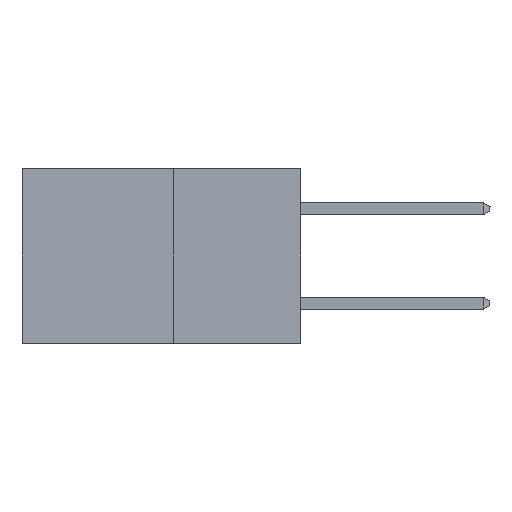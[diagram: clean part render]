
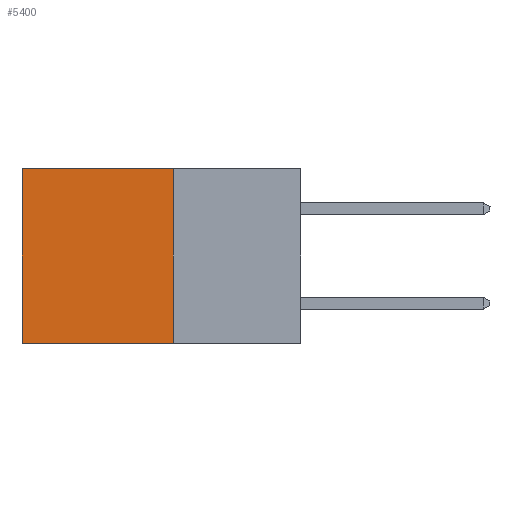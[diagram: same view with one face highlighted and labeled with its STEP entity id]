
A CAD part, left-side view. The second image highlights one B-rep face of the part: STEP entity #5400.
In plain terms, the highlighted planar face has unit normal (-1, 0, 0).
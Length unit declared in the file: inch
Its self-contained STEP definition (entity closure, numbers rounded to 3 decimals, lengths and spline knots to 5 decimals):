
#176 = CARTESIAN_POINT ( 'NONE',  ( 0.277, 0.27, -0.37 ) ) ;
#499 = CARTESIAN_POINT ( 'NONE',  ( 0.277, 0.59, -0.37 ) ) ;
#504 = FACE_OUTER_BOUND ( 'NONE', #11642, .T. ) ;
#892 = VECTOR ( 'NONE', #5699, 39.37008 ) ;
#1214 = VECTOR ( 'NONE', #12525, 39.37008 ) ;
#1572 = EDGE_CURVE ( 'NONE', #10851, #7207, #12171, .T. ) ;
#3573 = LINE ( 'NONE', #499, #892 ) ;
#3858 = CARTESIAN_POINT ( 'NONE',  ( 0.277, 0.27, -0.37 ) ) ;
#4150 = EDGE_CURVE ( 'NONE', #10851, #6409, #7095, .T. ) ;
#4247 = DIRECTION ( 'NONE',  ( 1., 0., 0. ) ) ;
#4442 = CARTESIAN_POINT ( 'NONE',  ( 0.277, 0.27, -0.37 ) ) ;
#4604 = DIRECTION ( 'NONE',  ( 0., 1., 0. ) ) ;
#4694 = EDGE_CURVE ( 'NONE', #6409, #11805, #8443, .T. ) ;
#4986 = ORIENTED_EDGE ( 'NONE', *, *, #4694, .F. ) ;
#5400 = ADVANCED_FACE ( 'NONE', ( #504 ), #7742, .F. ) ;
#5445 = CARTESIAN_POINT ( 'NONE',  ( 0.277, 0.59, -0.37 ) ) ;
#5451 = DIRECTION ( 'NONE',  ( 0., 0., -1. ) ) ;
#5509 = VECTOR ( 'NONE', #4604, 39.37008 ) ;
#5699 = DIRECTION ( 'NONE',  ( 0., 0., -1. ) ) ;
#6409 = VERTEX_POINT ( 'NONE', #3858 ) ;
#6990 = ORIENTED_EDGE ( 'NONE', *, *, #8558, .T. ) ;
#7095 = LINE ( 'NONE', #176, #1214 ) ;
#7135 = CARTESIAN_POINT ( 'NONE',  ( 0.277, 0.27, 0. ) ) ;
#7207 = VERTEX_POINT ( 'NONE', #9111 ) ;
#7601 = ORIENTED_EDGE ( 'NONE', *, *, #4150, .F. ) ;
#7668 = ORIENTED_EDGE ( 'NONE', *, *, #1572, .T. ) ;
#7682 = CARTESIAN_POINT ( 'NONE',  ( 0.277, 0.27, -0.37 ) ) ;
#7742 = PLANE ( 'NONE',  #9367 ) ;
#8443 = LINE ( 'NONE', #7682, #5509 ) ;
#8558 = EDGE_CURVE ( 'NONE', #7207, #11805, #3573, .T. ) ;
#9111 = CARTESIAN_POINT ( 'NONE',  ( 0.277, 0.59, 0. ) ) ;
#9367 = AXIS2_PLACEMENT_3D ( 'NONE', #4442, #4247, #5451 ) ;
#9725 = VECTOR ( 'NONE', #12225, 39.37008 ) ;
#10851 = VERTEX_POINT ( 'NONE', #7135 ) ;
#11642 = EDGE_LOOP ( 'NONE', ( #6990, #4986, #7601, #7668 ) ) ;
#11805 = VERTEX_POINT ( 'NONE', #5445 ) ;
#11907 = CARTESIAN_POINT ( 'NONE',  ( 0.277, 0.27, 0. ) ) ;
#12171 = LINE ( 'NONE', #11907, #9725 ) ;
#12225 = DIRECTION ( 'NONE',  ( 0., 1., 0. ) ) ;
#12525 = DIRECTION ( 'NONE',  ( 0., 0., -1. ) ) ;
